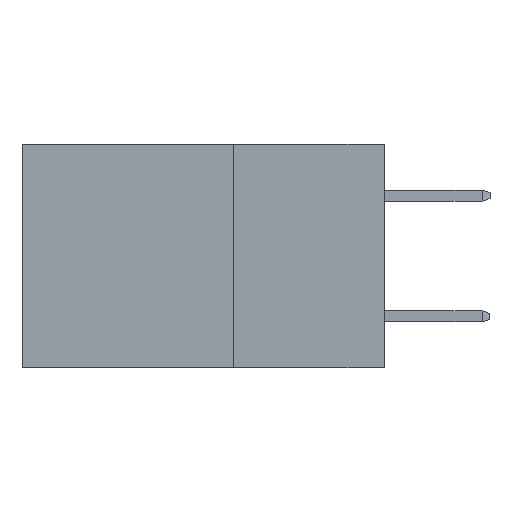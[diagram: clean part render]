
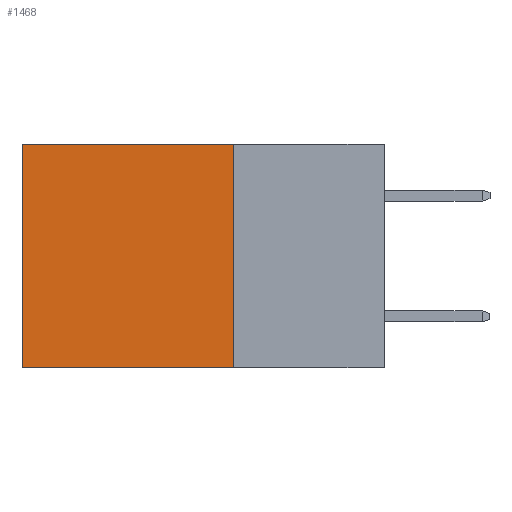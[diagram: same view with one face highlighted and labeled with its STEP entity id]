
A CAD part, left-side view. The second image highlights one B-rep face of the part: STEP entity #1468.
In plain terms, the highlighted planar face has unit normal (-1, 0, 0).
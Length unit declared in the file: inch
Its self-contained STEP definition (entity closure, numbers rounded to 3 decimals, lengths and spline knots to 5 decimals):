
#12 = EDGE_CURVE ( 'NONE', #5898, #209, #2554, .T. ) ;
#87 = DIRECTION ( 'NONE',  ( 0., 1., 0. ) ) ;
#209 = VERTEX_POINT ( 'NONE', #12219 ) ;
#1468 = ADVANCED_FACE ( 'NONE', ( #2693 ), #8005, .F. ) ;
#1496 = DIRECTION ( 'NONE',  ( 0., 0., -1. ) ) ;
#2414 = DIRECTION ( 'NONE',  ( 0., 0., -1. ) ) ;
#2554 = LINE ( 'NONE', #16041, #15606 ) ;
#2693 = FACE_OUTER_BOUND ( 'NONE', #11349, .T. ) ;
#3428 = CARTESIAN_POINT ( 'NONE',  ( 0.298, 0.6, -0.37 ) ) ;
#4279 = VERTEX_POINT ( 'NONE', #13608 ) ;
#5898 = VERTEX_POINT ( 'NONE', #14575 ) ;
#6219 = LINE ( 'NONE', #16328, #10026 ) ;
#7400 = ORIENTED_EDGE ( 'NONE', *, *, #14915, .T. ) ;
#7859 = CARTESIAN_POINT ( 'NONE',  ( 0.298, 0.6, 0. ) ) ;
#8005 = PLANE ( 'NONE',  #13083 ) ;
#8131 = VECTOR ( 'NONE', #1496, 39.37008 ) ;
#8543 = LINE ( 'NONE', #7859, #8131 ) ;
#8872 = ORIENTED_EDGE ( 'NONE', *, *, #12, .T. ) ;
#9882 = EDGE_CURVE ( 'NONE', #5898, #4279, #6219, .T. ) ;
#10026 = VECTOR ( 'NONE', #2414, 39.37008 ) ;
#10615 = CARTESIAN_POINT ( 'NONE',  ( 0.298, 0.25, -0.37 ) ) ;
#11069 = EDGE_CURVE ( 'NONE', #4279, #11342, #14851, .T. ) ;
#11342 = VERTEX_POINT ( 'NONE', #3428 ) ;
#11349 = EDGE_LOOP ( 'NONE', ( #7400, #12186, #15756, #8872 ) ) ;
#11539 = VECTOR ( 'NONE', #11834, 39.37008 ) ;
#11834 = DIRECTION ( 'NONE',  ( 0., 1., 0. ) ) ;
#12186 = ORIENTED_EDGE ( 'NONE', *, *, #11069, .F. ) ;
#12219 = CARTESIAN_POINT ( 'NONE',  ( 0.298, 0.6, 0. ) ) ;
#13083 = AXIS2_PLACEMENT_3D ( 'NONE', #15117, #15226, #15146 ) ;
#13608 = CARTESIAN_POINT ( 'NONE',  ( 0.298, 0.25, -0.37 ) ) ;
#14575 = CARTESIAN_POINT ( 'NONE',  ( 0.298, 0.25, 0. ) ) ;
#14851 = LINE ( 'NONE', #10615, #11539 ) ;
#14915 = EDGE_CURVE ( 'NONE', #209, #11342, #8543, .T. ) ;
#15117 = CARTESIAN_POINT ( 'NONE',  ( 0.298, 0.25, 0. ) ) ;
#15146 = DIRECTION ( 'NONE',  ( 0., 0., -1. ) ) ;
#15226 = DIRECTION ( 'NONE',  ( 1., 0., 0. ) ) ;
#15606 = VECTOR ( 'NONE', #87, 39.37008 ) ;
#15756 = ORIENTED_EDGE ( 'NONE', *, *, #9882, .F. ) ;
#16041 = CARTESIAN_POINT ( 'NONE',  ( 0.298, 0.25, 0. ) ) ;
#16328 = CARTESIAN_POINT ( 'NONE',  ( 0.298, 0.25, 0. ) ) ;
